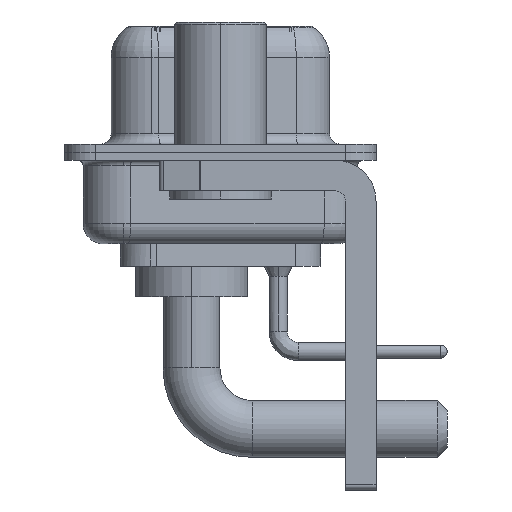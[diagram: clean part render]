
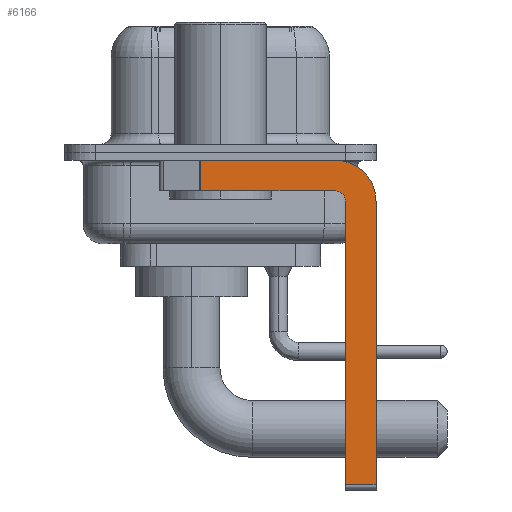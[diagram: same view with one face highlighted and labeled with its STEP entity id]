
A CAD part, left-side view. The second image highlights one B-rep face of the part: STEP entity #6166.
In plain terms, the highlighted planar face has unit normal (-1, 0, 0).
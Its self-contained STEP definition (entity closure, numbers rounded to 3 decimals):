
#3 = CARTESIAN_POINT ( 'NONE',  ( -2.9, -5.65, -16.35 ) ) ;
#364 = AXIS2_PLACEMENT_3D ( 'NONE', #23225, #12424, #6786 ) ;
#511 = CIRCLE ( 'NONE', #11657, 0.5 ) ;
#1073 = ORIENTED_EDGE ( 'NONE', *, *, #12237, .T. ) ;
#1142 = LINE ( 'NONE', #11968, #10915 ) ;
#1933 = LINE ( 'NONE', #12398, #12596 ) ;
#2173 = DIRECTION ( 'NONE',  ( 0., 1., 0. ) ) ;
#2337 = EDGE_CURVE ( 'NONE', #13391, #4794, #1933, .T. ) ;
#2604 = ORIENTED_EDGE ( 'NONE', *, *, #6591, .F. ) ;
#3440 = CARTESIAN_POINT ( 'NONE',  ( -2.9, -5.65, -0.4 ) ) ;
#4175 = CARTESIAN_POINT ( 'NONE',  ( -2.9, -7.65, -2.4 ) ) ;
#4501 = EDGE_CURVE ( 'NONE', #18686, #9615, #4518, .T. ) ;
#4518 = LINE ( 'NONE', #11732, #6677 ) ;
#4538 = EDGE_CURVE ( 'NONE', #19419, #11489, #1142, .T. ) ;
#4683 = ORIENTED_EDGE ( 'NONE', *, *, #16090, .F. ) ;
#4794 = VERTEX_POINT ( 'NONE', #14833 ) ;
#5344 = CARTESIAN_POINT ( 'NONE',  ( -2.9, 0.978, -1.9 ) ) ;
#5429 = ORIENTED_EDGE ( 'NONE', *, *, #4538, .F. ) ;
#6166 = ADVANCED_FACE ( 'NONE', ( #12788 ), #20107, .F. ) ;
#6591 = EDGE_CURVE ( 'NONE', #11489, #13391, #511, .T. ) ;
#6677 = VECTOR ( 'NONE', #21200, 1000. ) ;
#6752 = CARTESIAN_POINT ( 'NONE',  ( -2.9, -5.65, -2.4 ) ) ;
#6786 = DIRECTION ( 'NONE',  ( 0., 0., -1. ) ) ;
#7158 = DIRECTION ( 'NONE',  ( 0., 0., -1. ) ) ;
#7263 = DIRECTION ( 'NONE',  ( 0., 0., -1. ) ) ;
#7340 = EDGE_CURVE ( 'NONE', #22294, #4794, #9199, .T. ) ;
#8653 = CIRCLE ( 'NONE', #15942, 2. ) ;
#8809 = DIRECTION ( 'NONE',  ( 0., 0., 1. ) ) ;
#9062 = EDGE_LOOP ( 'NONE', ( #21543, #19781, #14094, #2604, #5429, #1073, #23095, #4683 ) ) ;
#9199 = LINE ( 'NONE', #5344, #22198 ) ;
#9615 = VERTEX_POINT ( 'NONE', #14316 ) ;
#9744 = DIRECTION ( 'NONE',  ( 0., -1., 0. ) ) ;
#10862 = VECTOR ( 'NONE', #20197, 1000. ) ;
#10915 = VECTOR ( 'NONE', #19394, 1000. ) ;
#11489 = VERTEX_POINT ( 'NONE', #17012 ) ;
#11657 = AXIS2_PLACEMENT_3D ( 'NONE', #6752, #14104, #8809 ) ;
#11675 = LINE ( 'NONE', #13730, #22032 ) ;
#11732 = CARTESIAN_POINT ( 'NONE',  ( -2.9, -7.65, -2.4 ) ) ;
#11858 = CARTESIAN_POINT ( 'NONE',  ( -2.9, -6.15, -16.35 ) ) ;
#11968 = CARTESIAN_POINT ( 'NONE',  ( -2.9, -6.15, -16.6 ) ) ;
#12237 = EDGE_CURVE ( 'NONE', #19419, #9615, #16107, .T. ) ;
#12398 = CARTESIAN_POINT ( 'NONE',  ( -2.9, -5.65, -1.9 ) ) ;
#12424 = DIRECTION ( 'NONE',  ( 1., 0., 0. ) ) ;
#12570 = DIRECTION ( 'NONE',  ( 1., 0., 0. ) ) ;
#12596 = VECTOR ( 'NONE', #2173, 1000. ) ;
#12788 = FACE_OUTER_BOUND ( 'NONE', #9062, .T. ) ;
#13391 = VERTEX_POINT ( 'NONE', #22576 ) ;
#13730 = CARTESIAN_POINT ( 'NONE',  ( -2.9, 3., -0.4 ) ) ;
#14094 = ORIENTED_EDGE ( 'NONE', *, *, #2337, .F. ) ;
#14104 = DIRECTION ( 'NONE',  ( -1., 0., 0. ) ) ;
#14307 = CARTESIAN_POINT ( 'NONE',  ( -2.9, 0.978, -0.4 ) ) ;
#14316 = CARTESIAN_POINT ( 'NONE',  ( -2.9, -7.65, -16.35 ) ) ;
#14833 = CARTESIAN_POINT ( 'NONE',  ( -2.9, 0.978, -1.9 ) ) ;
#15942 = AXIS2_PLACEMENT_3D ( 'NONE', #23459, #12570, #7158 ) ;
#16090 = EDGE_CURVE ( 'NONE', #17550, #18686, #8653, .T. ) ;
#16107 = LINE ( 'NONE', #3, #10862 ) ;
#17012 = CARTESIAN_POINT ( 'NONE',  ( -2.9, -6.15, -2.4 ) ) ;
#17550 = VERTEX_POINT ( 'NONE', #3440 ) ;
#18686 = VERTEX_POINT ( 'NONE', #4175 ) ;
#19394 = DIRECTION ( 'NONE',  ( 0., 0., 1. ) ) ;
#19419 = VERTEX_POINT ( 'NONE', #11858 ) ;
#19781 = ORIENTED_EDGE ( 'NONE', *, *, #7340, .T. ) ;
#20107 = PLANE ( 'NONE',  #364 ) ;
#20197 = DIRECTION ( 'NONE',  ( 0., -1., 0. ) ) ;
#20735 = EDGE_CURVE ( 'NONE', #22294, #17550, #11675, .T. ) ;
#21200 = DIRECTION ( 'NONE',  ( 0., 0., -1. ) ) ;
#21543 = ORIENTED_EDGE ( 'NONE', *, *, #20735, .F. ) ;
#22032 = VECTOR ( 'NONE', #9744, 1000. ) ;
#22198 = VECTOR ( 'NONE', #7263, 1000. ) ;
#22294 = VERTEX_POINT ( 'NONE', #14307 ) ;
#22576 = CARTESIAN_POINT ( 'NONE',  ( -2.9, -5.65, -1.9 ) ) ;
#23095 = ORIENTED_EDGE ( 'NONE', *, *, #4501, .F. ) ;
#23225 = CARTESIAN_POINT ( 'NONE',  ( -2.9, -5.65, -2.4 ) ) ;
#23459 = CARTESIAN_POINT ( 'NONE',  ( -2.9, -5.65, -2.4 ) ) ;
